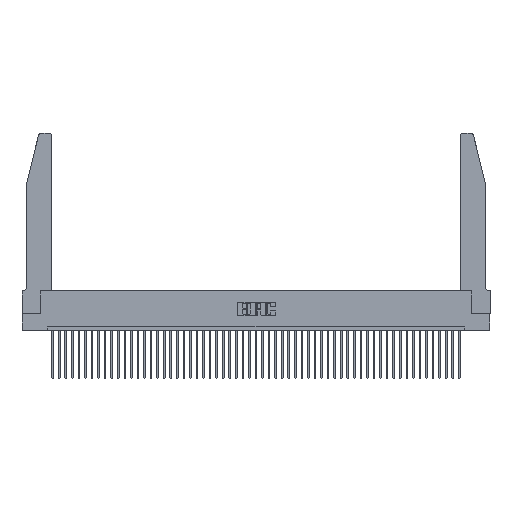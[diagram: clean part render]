
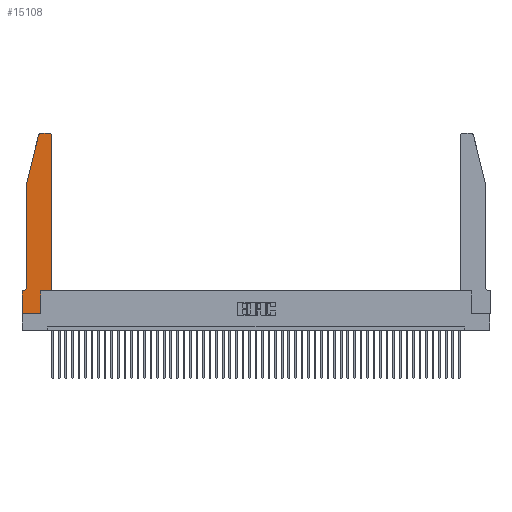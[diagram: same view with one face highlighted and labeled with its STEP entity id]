
A CAD part, top view. The second image highlights one B-rep face of the part: STEP entity #15108.
In plain terms, the highlighted planar face has unit normal (0, 0, 1).
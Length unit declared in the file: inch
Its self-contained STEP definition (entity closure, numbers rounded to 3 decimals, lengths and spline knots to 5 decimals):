
#1957 = CARTESIAN_POINT ( 'NONE',  ( 0.2865, 0., 0.37 ) ) ;
#2180 = DIRECTION ( 'NONE',  ( 0., -1., 0. ) ) ;
#2206 = CIRCLE ( 'NONE', #16272, 0.07 ) ;
#2847 = EDGE_CURVE ( 'NONE', #27235, #35231, #31836, .T. ) ;
#2969 = DIRECTION ( 'NONE',  ( 1., 0., 0. ) ) ;
#3131 = LINE ( 'NONE', #6984, #38295 ) ;
#3376 = DIRECTION ( 'NONE',  ( 0., 0., 1. ) ) ;
#3645 = CARTESIAN_POINT ( 'NONE',  ( 0.4505, 2.72, 0.37 ) ) ;
#3894 = CARTESIAN_POINT ( 'NONE',  ( 0.284, 2.75, 0.37 ) ) ;
#4979 = EDGE_CURVE ( 'NONE', #12479, #27667, #48353, .T. ) ;
#5310 = LINE ( 'NONE', #37598, #34587 ) ;
#5326 = AXIS2_PLACEMENT_3D ( 'NONE', #12817, #24312, #47990 ) ;
#6403 = ORIENTED_EDGE ( 'NONE', *, *, #2847, .T. ) ;
#6984 = CARTESIAN_POINT ( 'NONE',  ( 0., 0., 0.37 ) ) ;
#7586 = EDGE_CURVE ( 'NONE', #35231, #15679, #2206, .T. ) ;
#8047 = CARTESIAN_POINT ( 'NONE',  ( 0., 0.35, 0.37 ) ) ;
#8697 = CIRCLE ( 'NONE', #28366, 0.03 ) ;
#9061 = CARTESIAN_POINT ( 'NONE',  ( 0.4505, 0.35, 0.37 ) ) ;
#9064 = ORIENTED_EDGE ( 'NONE', *, *, #43100, .T. ) ;
#11125 = VERTEX_POINT ( 'NONE', #23943 ) ;
#11564 = VECTOR ( 'NONE', #2180, 39.37008 ) ;
#12145 = EDGE_CURVE ( 'NONE', #26170, #17840, #5310, .T. ) ;
#12479 = VERTEX_POINT ( 'NONE', #36246 ) ;
#12817 = CARTESIAN_POINT ( 'NONE',  ( 0., 0.35, 0.37 ) ) ;
#13300 = EDGE_CURVE ( 'NONE', #18569, #27235, #22599, .T. ) ;
#13465 = ORIENTED_EDGE ( 'NONE', *, *, #4979, .T. ) ;
#15108 = ADVANCED_FACE ( 'NONE', ( #23592 ), #24995, .T. ) ;
#15505 = CARTESIAN_POINT ( 'NONE',  ( 0.4505, 0.35, 0.37 ) ) ;
#15679 = VERTEX_POINT ( 'NONE', #24352 ) ;
#16272 = AXIS2_PLACEMENT_3D ( 'NONE', #47942, #44448, #33345 ) ;
#16284 = CARTESIAN_POINT ( 'NONE',  ( 0.0755, 2., 0.37 ) ) ;
#16375 = VECTOR ( 'NONE', #43668, 39.37008 ) ;
#16683 = CARTESIAN_POINT ( 'NONE',  ( 0.0755, 2., 0.37 ) ) ;
#16974 = CARTESIAN_POINT ( 'NONE',  ( 0.2865, 0.35, 0.37 ) ) ;
#17079 = ORIENTED_EDGE ( 'NONE', *, *, #13300, .T. ) ;
#17790 = CARTESIAN_POINT ( 'NONE',  ( 0.284, 2.72, 0.37 ) ) ;
#17840 = VERTEX_POINT ( 'NONE', #26735 ) ;
#17888 = DIRECTION ( 'NONE',  ( 0., 1., 0. ) ) ;
#18569 = VERTEX_POINT ( 'NONE', #35056 ) ;
#20250 = VERTEX_POINT ( 'NONE', #3645 ) ;
#20689 = ORIENTED_EDGE ( 'NONE', *, *, #49073, .T. ) ;
#20760 = VECTOR ( 'NONE', #34644, 39.37008 ) ;
#22544 = DIRECTION ( 'NONE',  ( 1., 0., 0. ) ) ;
#22599 = LINE ( 'NONE', #34046, #20760 ) ;
#23592 = FACE_OUTER_BOUND ( 'NONE', #48949, .T. ) ;
#23943 = CARTESIAN_POINT ( 'NONE',  ( 0.4205, 2.75, 0.37 ) ) ;
#24312 = DIRECTION ( 'NONE',  ( 0., 0., 1. ) ) ;
#24352 = CARTESIAN_POINT ( 'NONE',  ( 0.0055, 0.35, 0.37 ) ) ;
#24743 = EDGE_CURVE ( 'NONE', #20250, #11125, #8697, .T. ) ;
#24995 = PLANE ( 'NONE',  #5326 ) ;
#25103 = CARTESIAN_POINT ( 'NONE',  ( 0.0755, 0.35, 0.37 ) ) ;
#26170 = VERTEX_POINT ( 'NONE', #8047 ) ;
#26215 = CARTESIAN_POINT ( 'NONE',  ( 0.4205, 2.72, 0.37 ) ) ;
#26558 = LINE ( 'NONE', #16974, #16375 ) ;
#26735 = CARTESIAN_POINT ( 'NONE',  ( 0., 0., 0.37 ) ) ;
#26743 = ORIENTED_EDGE ( 'NONE', *, *, #12145, .T. ) ;
#27235 = VERTEX_POINT ( 'NONE', #16284 ) ;
#27309 = AXIS2_PLACEMENT_3D ( 'NONE', #17790, #29824, #2969 ) ;
#27667 = VERTEX_POINT ( 'NONE', #9061 ) ;
#27887 = VECTOR ( 'NONE', #48606, 39.37008 ) ;
#28366 = AXIS2_PLACEMENT_3D ( 'NONE', #26215, #3376, #22544 ) ;
#29824 = DIRECTION ( 'NONE',  ( 0., 0., 1. ) ) ;
#30770 = ORIENTED_EDGE ( 'NONE', *, *, #24743, .T. ) ;
#31836 = LINE ( 'NONE', #16683, #11564 ) ;
#32122 = EDGE_CURVE ( 'NONE', #27667, #20250, #39020, .T. ) ;
#32882 = EDGE_CURVE ( 'NONE', #17840, #33235, #3131, .T. ) ;
#33193 = ORIENTED_EDGE ( 'NONE', *, *, #42378, .T. ) ;
#33235 = VERTEX_POINT ( 'NONE', #1957 ) ;
#33283 = DIRECTION ( 'NONE',  ( 0., -1., 0. ) ) ;
#33345 = DIRECTION ( 'NONE',  ( -1., 0., 0. ) ) ;
#33949 = ORIENTED_EDGE ( 'NONE', *, *, #7586, .T. ) ;
#34046 = CARTESIAN_POINT ( 'NONE',  ( 0.0755, 2., 0.37 ) ) ;
#34541 = ORIENTED_EDGE ( 'NONE', *, *, #45617, .T. ) ;
#34587 = VECTOR ( 'NONE', #33283, 39.37008 ) ;
#34644 = DIRECTION ( 'NONE',  ( -0.239, -0.971, 0. ) ) ;
#35056 = CARTESIAN_POINT ( 'NONE',  ( 0.25487, 2.72718, 0.37 ) ) ;
#35231 = VERTEX_POINT ( 'NONE', #43083 ) ;
#36246 = CARTESIAN_POINT ( 'NONE',  ( 0.2865, 0.35, 0.37 ) ) ;
#37598 = CARTESIAN_POINT ( 'NONE',  ( 0., 0., 0.37 ) ) ;
#38295 = VECTOR ( 'NONE', #48638, 39.37008 ) ;
#38587 = ORIENTED_EDGE ( 'NONE', *, *, #32882, .T. ) ;
#38618 = LINE ( 'NONE', #44602, #27887 ) ;
#39020 = LINE ( 'NONE', #15505, #40852 ) ;
#39074 = CIRCLE ( 'NONE', #27309, 0.03 ) ;
#39764 = VERTEX_POINT ( 'NONE', #3894 ) ;
#40444 = DIRECTION ( 'NONE',  ( -1., 0., 0. ) ) ;
#40852 = VECTOR ( 'NONE', #17888, 39.37008 ) ;
#41216 = CARTESIAN_POINT ( 'NONE',  ( 0.4505, 0.35, 0.37 ) ) ;
#42018 = ORIENTED_EDGE ( 'NONE', *, *, #32122, .T. ) ;
#42378 = EDGE_CURVE ( 'NONE', #39764, #18569, #39074, .T. ) ;
#43083 = CARTESIAN_POINT ( 'NONE',  ( 0.0755, 0.42, 0.37 ) ) ;
#43100 = EDGE_CURVE ( 'NONE', #33235, #12479, #26558, .T. ) ;
#43668 = DIRECTION ( 'NONE',  ( 0., 1., 0. ) ) ;
#44173 = VECTOR ( 'NONE', #49037, 39.37008 ) ;
#44448 = DIRECTION ( 'NONE',  ( 0., 0., -1. ) ) ;
#44602 = CARTESIAN_POINT ( 'NONE',  ( 0.2605, 2.75, 0.37 ) ) ;
#45511 = VECTOR ( 'NONE', #40444, 39.37008 ) ;
#45617 = EDGE_CURVE ( 'NONE', #15679, #26170, #49134, .T. ) ;
#47942 = CARTESIAN_POINT ( 'NONE',  ( 0.0055, 0.42, 0.37 ) ) ;
#47990 = DIRECTION ( 'NONE',  ( 1., 0., 0. ) ) ;
#48353 = LINE ( 'NONE', #41216, #44173 ) ;
#48606 = DIRECTION ( 'NONE',  ( -1., 0., 0. ) ) ;
#48638 = DIRECTION ( 'NONE',  ( 1., 0., 0. ) ) ;
#48949 = EDGE_LOOP ( 'NONE', ( #20689, #33193, #17079, #6403, #33949, #34541, #26743, #38587, #9064, #13465, #42018, #30770 ) ) ;
#49037 = DIRECTION ( 'NONE',  ( 1., 0., 0. ) ) ;
#49073 = EDGE_CURVE ( 'NONE', #11125, #39764, #38618, .T. ) ;
#49134 = LINE ( 'NONE', #25103, #45511 ) ;
